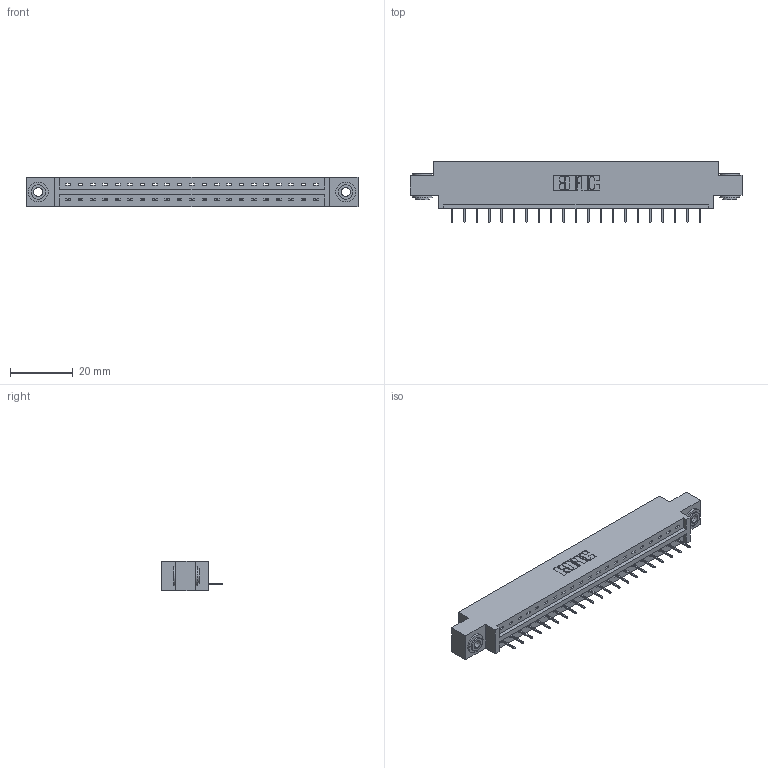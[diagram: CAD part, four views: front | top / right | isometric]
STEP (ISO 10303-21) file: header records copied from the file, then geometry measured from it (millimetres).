
FILE_DESCRIPTION (( 'STEP AP203' ), '1' );
FILE_NAME ('387-021-524-603.STEP', '2018-09-14T01:44:58', ( '' ), ( '' ), 'SwSTEP 2.0', 'SolidWorks 2016', '' );
FILE_SCHEMA (( 'CONFIG_CONTROL_DESIGN' ));
Length unit declared in the file: inch
Products named in the file (4): 337 Part_0.170 Offset - 0.156 Dia-TH; 345-292-001_345-293-124; 345-250-002_345-250-002-102; 387-021-524-603
Assembly tree (24 placements, depth 2):
  387-021-524-603
    337 Part_0.170 Offset - 0.156 Dia-TH
    345-292-001_345-293-124  x21
    345-250-002_345-250-002-102  x2
Bounding box: 106.22 x 19.69 x 9.4 mm (x, y, z)
Volume: 10596.2 mm3; surface area: 10870.5 mm2
Topology: 24 solids, 24 shells, 1542 faces, 4431 edges, 2866 vertices
Faces by surface type: plane 1176, cylinder 358, cone 8
Entity records: 19182 total; most frequent: CARTESIAN_POINT 3316, ORIENTED_EDGE 3266, DIRECTION 2869, EDGE_CURVE 1633, VECTOR 1485, LINE 1485, VERTEX_POINT 1082, AXIS2_PLACEMENT_3D 692
